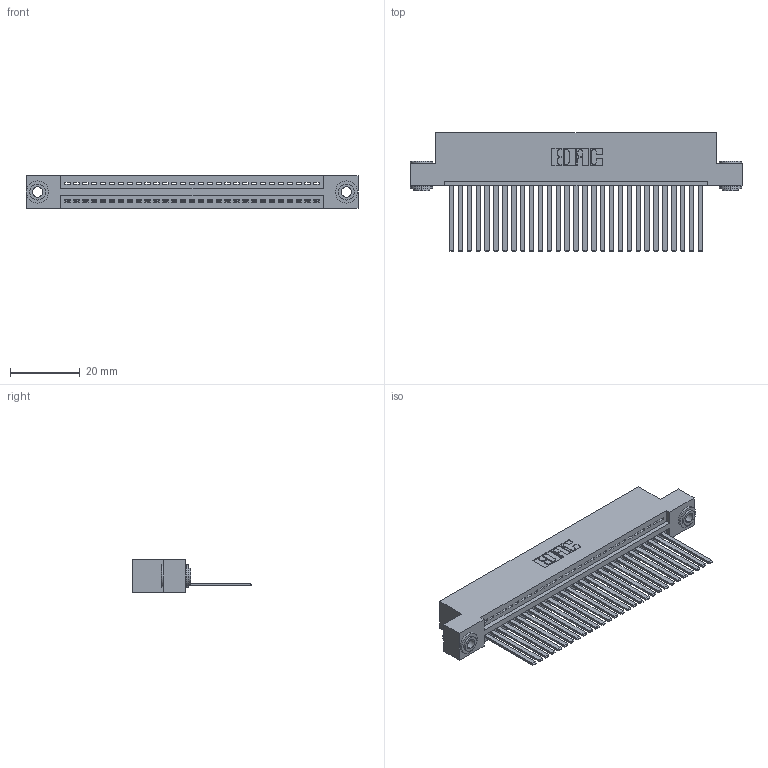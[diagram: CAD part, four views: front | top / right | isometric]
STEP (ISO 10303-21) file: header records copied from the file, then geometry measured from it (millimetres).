
FILE_DESCRIPTION (( 'STEP AP203' ), '1' );
FILE_NAME ('345-029-544-103.STEP', '2019-10-07T08:14:49', ( '' ), ( '' ), 'SwSTEP 2.0', 'SolidWorks 2016', '' );
FILE_SCHEMA (( 'CONFIG_CONTROL_DESIGN' ));
Length unit declared in the file: inch
Products named in the file (4): 345-029-544-103; 345-250-002_345-250-002-102; 345 Part_Flush Mounting Lugs - 0.156 Dia-TH; 345-292-001_345-293-144
Assembly tree (32 placements, depth 2):
  345-029-544-103
    345 Part_Flush Mounting Lugs - 0.156 Dia-TH
    345-292-001_345-293-144  x29
    345-250-002_345-250-002-102  x2
Bounding box: 94.87 x 33.96 x 9.4 mm (x, y, z)
Volume: 9259.5 mm3; surface area: 13351.1 mm2
Topology: 32 solids, 32 shells, 1672 faces, 4999 edges, 3290 vertices
Faces by surface type: plane 1134, cylinder 530, cone 8
Entity records: 24042 total; most frequent: CARTESIAN_POINT 4142, ORIENTED_EDGE 4098, DIRECTION 3665, EDGE_CURVE 2049, VECTOR 1781, LINE 1781, VERTEX_POINT 1362, AXIS2_PLACEMENT_3D 942
